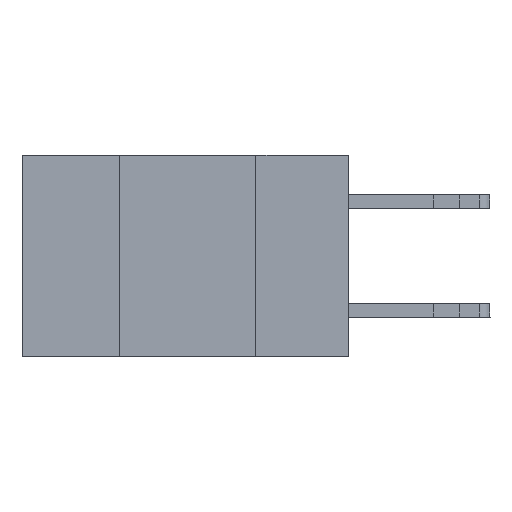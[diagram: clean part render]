
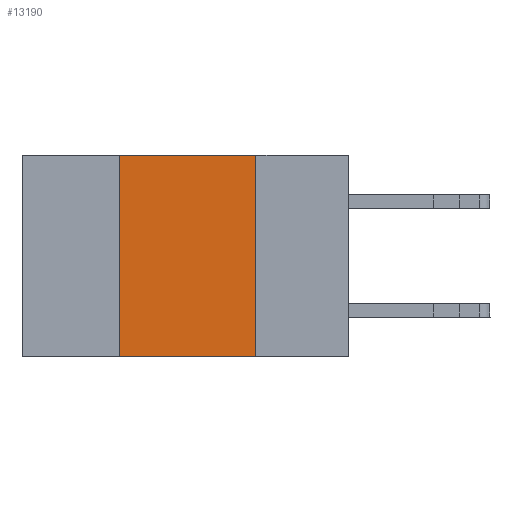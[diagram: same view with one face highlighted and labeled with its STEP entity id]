
A CAD part, left-side view. The second image highlights one B-rep face of the part: STEP entity #13190.
In plain terms, the highlighted planar face has unit normal (-1, 0, 0).
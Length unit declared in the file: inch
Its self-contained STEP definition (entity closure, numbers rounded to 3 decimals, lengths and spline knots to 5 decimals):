
#22 = ORIENTED_EDGE ( 'NONE', *, *, #3260, .F. ) ;
#324 = DIRECTION ( 'NONE',  ( 0., 0., 1. ) ) ;
#834 = VERTEX_POINT ( 'NONE', #15615 ) ;
#1220 = ORIENTED_EDGE ( 'NONE', *, *, #11122, .F. ) ;
#3260 = EDGE_CURVE ( 'NONE', #19275, #7593, #21467, .T. ) ;
#4347 = CARTESIAN_POINT ( 'NONE',  ( 0., 0.6, 0. ) ) ;
#5999 = CARTESIAN_POINT ( 'NONE',  ( 0., 0.17, 0. ) ) ;
#6236 = DIRECTION ( 'NONE',  ( 0., 0., -1. ) ) ;
#6397 = CARTESIAN_POINT ( 'NONE',  ( 0., 0.42, 0. ) ) ;
#6493 = VECTOR ( 'NONE', #19141, 39.37008 ) ;
#7037 = CARTESIAN_POINT ( 'NONE',  ( 0., 0.17, 0. ) ) ;
#7593 = VERTEX_POINT ( 'NONE', #7037 ) ;
#8546 = VECTOR ( 'NONE', #324, 39.37008 ) ;
#9056 = LINE ( 'NONE', #22704, #23917 ) ;
#9480 = FACE_OUTER_BOUND ( 'NONE', #17261, .T. ) ;
#9741 = CARTESIAN_POINT ( 'NONE',  ( 0., 0.42, 0. ) ) ;
#9860 = EDGE_CURVE ( 'NONE', #7593, #834, #20857, .T. ) ;
#11122 = EDGE_CURVE ( 'NONE', #15103, #19275, #17969, .T. ) ;
#11838 = ORIENTED_EDGE ( 'NONE', *, *, #12396, .T. ) ;
#12396 = EDGE_CURVE ( 'NONE', #15103, #834, #9056, .T. ) ;
#13190 = ADVANCED_FACE ( 'NONE', ( #9480 ), #15635, .F. ) ;
#15081 = ORIENTED_EDGE ( 'NONE', *, *, #9860, .F. ) ;
#15103 = VERTEX_POINT ( 'NONE', #19713 ) ;
#15332 = DIRECTION ( 'NONE',  ( 0., -1., 0. ) ) ;
#15615 = CARTESIAN_POINT ( 'NONE',  ( 0., 0.17, -0.37 ) ) ;
#15635 = PLANE ( 'NONE',  #22274 ) ;
#17113 = CARTESIAN_POINT ( 'NONE',  ( 0., 0.6, 0. ) ) ;
#17261 = EDGE_LOOP ( 'NONE', ( #15081, #22, #1220, #11838 ) ) ;
#17520 = DIRECTION ( 'NONE',  ( 1., 0., 0. ) ) ;
#17969 = LINE ( 'NONE', #9741, #8546 ) ;
#19141 = DIRECTION ( 'NONE',  ( 0., 0., -1. ) ) ;
#19275 = VERTEX_POINT ( 'NONE', #6397 ) ;
#19713 = CARTESIAN_POINT ( 'NONE',  ( 0., 0.42, -0.37 ) ) ;
#20857 = LINE ( 'NONE', #5999, #6493 ) ;
#20889 = VECTOR ( 'NONE', #24039, 39.37008 ) ;
#21467 = LINE ( 'NONE', #17113, #20889 ) ;
#22274 = AXIS2_PLACEMENT_3D ( 'NONE', #4347, #17520, #6236 ) ;
#22704 = CARTESIAN_POINT ( 'NONE',  ( 0., 0.6, -0.37 ) ) ;
#23917 = VECTOR ( 'NONE', #15332, 39.37008 ) ;
#24039 = DIRECTION ( 'NONE',  ( 0., -1., 0. ) ) ;
